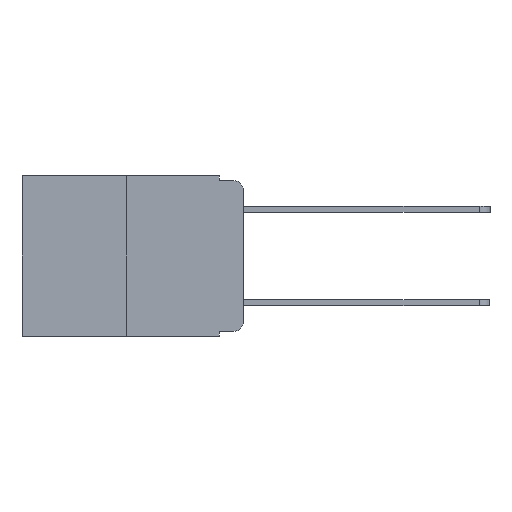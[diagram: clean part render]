
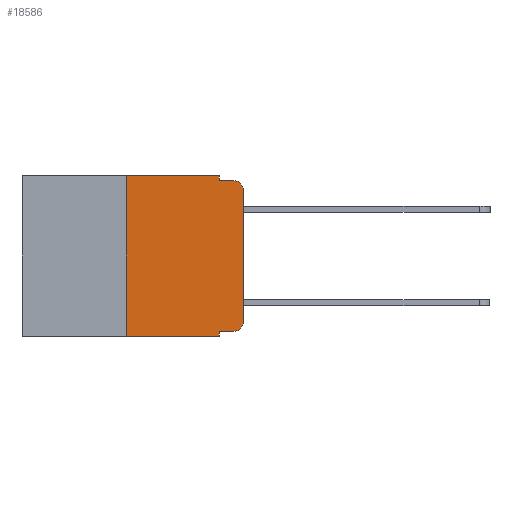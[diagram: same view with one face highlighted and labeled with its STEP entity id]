
A CAD part, left-side view. The second image highlights one B-rep face of the part: STEP entity #18586.
In plain terms, the highlighted planar face has unit normal (-1, 0, 0).
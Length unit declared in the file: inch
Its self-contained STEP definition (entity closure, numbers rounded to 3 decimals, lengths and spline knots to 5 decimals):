
#71 = CARTESIAN_POINT ( 'NONE',  ( 0., 0.051, 0. ) ) ;
#416 = CARTESIAN_POINT ( 'NONE',  ( 0., 0.051, -0.01 ) ) ;
#998 = EDGE_CURVE ( 'NONE', #21214, #10398, #20926, .T. ) ;
#1653 = ORIENTED_EDGE ( 'NONE', *, *, #5741, .T. ) ;
#1965 = CARTESIAN_POINT ( 'NONE',  ( 0., 0.25, 0. ) ) ;
#2157 = DIRECTION ( 'NONE',  ( 1., 0., 0. ) ) ;
#2608 = CARTESIAN_POINT ( 'NONE',  ( 0., 0.051, -0.333 ) ) ;
#3365 = VERTEX_POINT ( 'NONE', #20950 ) ;
#3992 = PLANE ( 'NONE',  #14650 ) ;
#4342 = CARTESIAN_POINT ( 'NONE',  ( 0., 0.473, -0.343 ) ) ;
#4402 = CARTESIAN_POINT ( 'NONE',  ( 0., 0.02, -0.313 ) ) ;
#4405 = ORIENTED_EDGE ( 'NONE', *, *, #16468, .F. ) ;
#4960 = LINE ( 'NONE', #13569, #23463 ) ;
#5452 = VERTEX_POINT ( 'NONE', #17955 ) ;
#5576 = ORIENTED_EDGE ( 'NONE', *, *, #5911, .T. ) ;
#5741 = EDGE_CURVE ( 'NONE', #3365, #10626, #21650, .T. ) ;
#5770 = EDGE_LOOP ( 'NONE', ( #5576, #6049, #4405, #14841, #8483, #12315, #5806, #13531, #11203, #1653 ) ) ;
#5806 = ORIENTED_EDGE ( 'NONE', *, *, #23132, .T. ) ;
#5911 = EDGE_CURVE ( 'NONE', #10626, #6657, #13605, .T. ) ;
#5920 = VECTOR ( 'NONE', #21870, 39.37008 ) ;
#6012 = EDGE_CURVE ( 'NONE', #10398, #19585, #16072, .T. ) ;
#6049 = ORIENTED_EDGE ( 'NONE', *, *, #22436, .T. ) ;
#6067 = EDGE_CURVE ( 'NONE', #19585, #6173, #20239, .T. ) ;
#6173 = VERTEX_POINT ( 'NONE', #416 ) ;
#6263 = VERTEX_POINT ( 'NONE', #2608 ) ;
#6281 = DIRECTION ( 'NONE',  ( 0., 0., -1. ) ) ;
#6624 = VECTOR ( 'NONE', #9961, 39.37008 ) ;
#6657 = VERTEX_POINT ( 'NONE', #18249 ) ;
#6790 = VECTOR ( 'NONE', #18071, 39.37008 ) ;
#7179 = DIRECTION ( 'NONE',  ( 0., 0., 1. ) ) ;
#8073 = CARTESIAN_POINT ( 'NONE',  ( 0., 0.25, 0. ) ) ;
#8483 = ORIENTED_EDGE ( 'NONE', *, *, #6012, .F. ) ;
#8757 = CARTESIAN_POINT ( 'NONE',  ( 0., 0.051, -0.01 ) ) ;
#8784 = VECTOR ( 'NONE', #7179, 39.37008 ) ;
#9507 = VERTEX_POINT ( 'NONE', #14077 ) ;
#9729 = CARTESIAN_POINT ( 'NONE',  ( 0., 0.02, -0.03 ) ) ;
#9961 = DIRECTION ( 'NONE',  ( 0., 0., 1. ) ) ;
#10398 = VERTEX_POINT ( 'NONE', #1965 ) ;
#10626 = VERTEX_POINT ( 'NONE', #18901 ) ;
#10732 = LINE ( 'NONE', #4342, #19664 ) ;
#11203 = ORIENTED_EDGE ( 'NONE', *, *, #13020, .T. ) ;
#11261 = CARTESIAN_POINT ( 'NONE',  ( 0., 0.473, 0. ) ) ;
#11314 = VECTOR ( 'NONE', #11461, 39.37008 ) ;
#11461 = DIRECTION ( 'NONE',  ( 0., -1., 0. ) ) ;
#11550 = DIRECTION ( 'NONE',  ( 0., 0., -1. ) ) ;
#11689 = VECTOR ( 'NONE', #21265, 39.37008 ) ;
#12315 = ORIENTED_EDGE ( 'NONE', *, *, #998, .F. ) ;
#12345 = CARTESIAN_POINT ( 'NONE',  ( 0., 0.051, 0. ) ) ;
#12717 = CARTESIAN_POINT ( 'NONE',  ( 0., 0.051, 0. ) ) ;
#12746 = CIRCLE ( 'NONE', #15170, 0.02 ) ;
#13020 = EDGE_CURVE ( 'NONE', #6263, #3365, #4960, .T. ) ;
#13438 = DIRECTION ( 'NONE',  ( 0., -1., 0. ) ) ;
#13531 = ORIENTED_EDGE ( 'NONE', *, *, #17772, .F. ) ;
#13569 = CARTESIAN_POINT ( 'NONE',  ( 0., 0.051, -0.333 ) ) ;
#13605 = LINE ( 'NONE', #23253, #8784 ) ;
#13782 = AXIS2_PLACEMENT_3D ( 'NONE', #4402, #17041, #6281 ) ;
#14077 = CARTESIAN_POINT ( 'NONE',  ( 0., 0.051, -0.343 ) ) ;
#14650 = AXIS2_PLACEMENT_3D ( 'NONE', #11261, #2157, #14952 ) ;
#14841 = ORIENTED_EDGE ( 'NONE', *, *, #6067, .F. ) ;
#14952 = DIRECTION ( 'NONE',  ( 0., 0., -1. ) ) ;
#15170 = AXIS2_PLACEMENT_3D ( 'NONE', #9729, #22230, #11550 ) ;
#15354 = DIRECTION ( 'NONE',  ( 0., -1., 0. ) ) ;
#16072 = LINE ( 'NONE', #16439, #11314 ) ;
#16345 = LINE ( 'NONE', #12717, #6790 ) ;
#16439 = CARTESIAN_POINT ( 'NONE',  ( 0., 0.473, 0. ) ) ;
#16468 = EDGE_CURVE ( 'NONE', #6173, #5452, #20595, .T. ) ;
#17041 = DIRECTION ( 'NONE',  ( -1., 0., 0. ) ) ;
#17772 = EDGE_CURVE ( 'NONE', #6263, #9507, #16345, .T. ) ;
#17955 = CARTESIAN_POINT ( 'NONE',  ( 0., 0.02, -0.01 ) ) ;
#18071 = DIRECTION ( 'NONE',  ( 0., 0., -1. ) ) ;
#18249 = CARTESIAN_POINT ( 'NONE',  ( 0., 0., -0.03 ) ) ;
#18534 = FACE_OUTER_BOUND ( 'NONE', #5770, .T. ) ;
#18586 = ADVANCED_FACE ( 'NONE', ( #18534 ), #3992, .F. ) ;
#18901 = CARTESIAN_POINT ( 'NONE',  ( 0., 0., -0.313 ) ) ;
#19585 = VERTEX_POINT ( 'NONE', #12345 ) ;
#19664 = VECTOR ( 'NONE', #13438, 39.37008 ) ;
#20239 = LINE ( 'NONE', #71, #5920 ) ;
#20595 = LINE ( 'NONE', #8757, #11689 ) ;
#20926 = LINE ( 'NONE', #8073, #6624 ) ;
#20950 = CARTESIAN_POINT ( 'NONE',  ( 0., 0.02, -0.333 ) ) ;
#21214 = VERTEX_POINT ( 'NONE', #21649 ) ;
#21265 = DIRECTION ( 'NONE',  ( 0., -1., 0. ) ) ;
#21649 = CARTESIAN_POINT ( 'NONE',  ( 0., 0.25, -0.343 ) ) ;
#21650 = CIRCLE ( 'NONE', #13782, 0.02 ) ;
#21870 = DIRECTION ( 'NONE',  ( 0., 0., -1. ) ) ;
#22230 = DIRECTION ( 'NONE',  ( -1., 0., 0. ) ) ;
#22436 = EDGE_CURVE ( 'NONE', #6657, #5452, #12746, .T. ) ;
#23132 = EDGE_CURVE ( 'NONE', #21214, #9507, #10732, .T. ) ;
#23253 = CARTESIAN_POINT ( 'NONE',  ( 0., 0., 0. ) ) ;
#23463 = VECTOR ( 'NONE', #15354, 39.37008 ) ;
